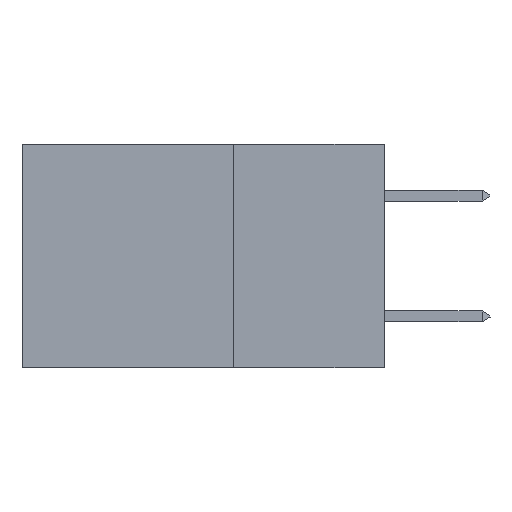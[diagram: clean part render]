
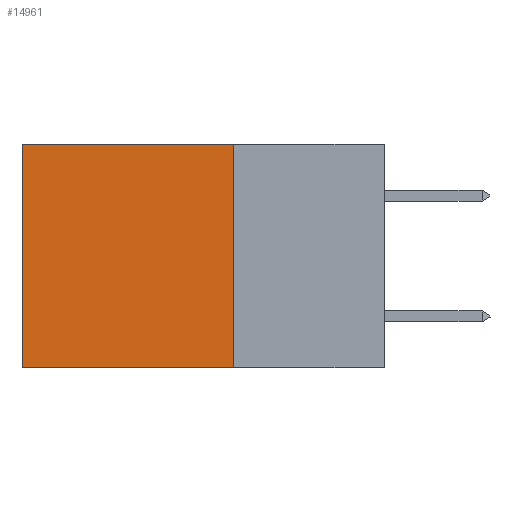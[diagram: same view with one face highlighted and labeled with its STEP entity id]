
A CAD part, left-side view. The second image highlights one B-rep face of the part: STEP entity #14961.
In plain terms, the highlighted planar face has unit normal (-1, 0, 0).
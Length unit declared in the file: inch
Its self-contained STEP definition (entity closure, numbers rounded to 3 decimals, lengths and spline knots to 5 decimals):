
#87 = EDGE_CURVE ( 'NONE', #13557, #3487, #24519, .T. ) ;
#647 = CARTESIAN_POINT ( 'NONE',  ( 0.2875, 0.25, -0.37 ) ) ;
#1146 = EDGE_CURVE ( 'NONE', #13557, #1900, #7943, .T. ) ;
#1178 = EDGE_CURVE ( 'NONE', #1900, #15284, #20401, .T. ) ;
#1626 = DIRECTION ( 'NONE',  ( 0., 1., 0. ) ) ;
#1900 = VERTEX_POINT ( 'NONE', #27846 ) ;
#3215 = VECTOR ( 'NONE', #19741, 39.37008 ) ;
#3302 = DIRECTION ( 'NONE',  ( 0., 0., -1. ) ) ;
#3487 = VERTEX_POINT ( 'NONE', #647 ) ;
#3783 = CARTESIAN_POINT ( 'NONE',  ( 0.2875, 0.25, -0.37 ) ) ;
#4682 = CARTESIAN_POINT ( 'NONE',  ( 0.2875, 0.25, 0. ) ) ;
#5015 = FACE_OUTER_BOUND ( 'NONE', #13851, .T. ) ;
#5528 = CARTESIAN_POINT ( 'NONE',  ( 0.2875, 0.25, 0. ) ) ;
#6067 = ORIENTED_EDGE ( 'NONE', *, *, #1146, .T. ) ;
#7678 = VECTOR ( 'NONE', #3302, 39.37008 ) ;
#7943 = LINE ( 'NONE', #14941, #12310 ) ;
#9669 = AXIS2_PLACEMENT_3D ( 'NONE', #4682, #17312, #11195 ) ;
#10710 = DIRECTION ( 'NONE',  ( 0., 1., 0. ) ) ;
#11116 = ORIENTED_EDGE ( 'NONE', *, *, #1178, .T. ) ;
#11195 = DIRECTION ( 'NONE',  ( 0., 0., -1. ) ) ;
#12221 = ORIENTED_EDGE ( 'NONE', *, *, #87, .F. ) ;
#12310 = VECTOR ( 'NONE', #10710, 39.37008 ) ;
#12913 = EDGE_CURVE ( 'NONE', #3487, #15284, #23953, .T. ) ;
#13557 = VERTEX_POINT ( 'NONE', #23135 ) ;
#13851 = EDGE_LOOP ( 'NONE', ( #11116, #16150, #12221, #6067 ) ) ;
#14941 = CARTESIAN_POINT ( 'NONE',  ( 0.2875, 0.25, 0. ) ) ;
#14961 = ADVANCED_FACE ( 'NONE', ( #5015 ), #17580, .F. ) ;
#15284 = VERTEX_POINT ( 'NONE', #24833 ) ;
#16150 = ORIENTED_EDGE ( 'NONE', *, *, #12913, .F. ) ;
#17312 = DIRECTION ( 'NONE',  ( 1., 0., 0. ) ) ;
#17580 = PLANE ( 'NONE',  #9669 ) ;
#19741 = DIRECTION ( 'NONE',  ( 0., 0., -1. ) ) ;
#20401 = LINE ( 'NONE', #23491, #3215 ) ;
#21278 = VECTOR ( 'NONE', #1626, 39.37008 ) ;
#23135 = CARTESIAN_POINT ( 'NONE',  ( 0.2875, 0.25, 0. ) ) ;
#23491 = CARTESIAN_POINT ( 'NONE',  ( 0.2875, 0.6, 0. ) ) ;
#23953 = LINE ( 'NONE', #3783, #21278 ) ;
#24519 = LINE ( 'NONE', #5528, #7678 ) ;
#24833 = CARTESIAN_POINT ( 'NONE',  ( 0.2875, 0.6, -0.37 ) ) ;
#27846 = CARTESIAN_POINT ( 'NONE',  ( 0.2875, 0.6, 0. ) ) ;
